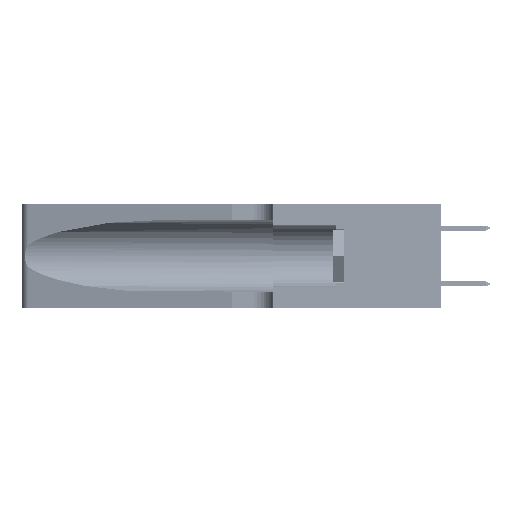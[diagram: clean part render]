
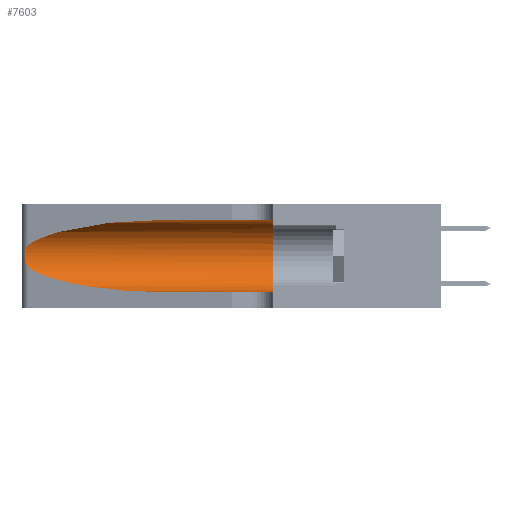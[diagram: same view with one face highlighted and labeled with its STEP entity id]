
A CAD part, left-side view. The second image highlights one B-rep face of the part: STEP entity #7603.
In plain terms, the highlighted cylindrical face has radius 3.308 mm (diameter 6.617 mm), a partial arc.
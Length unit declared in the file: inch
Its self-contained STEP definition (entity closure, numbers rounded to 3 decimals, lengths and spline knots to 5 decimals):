
#663 = EDGE_CURVE ( 'NONE', #46274, #41086, #32545, .T. ) ;
#688 = VERTEX_POINT ( 'NONE', #49093 ) ;
#1128 = VECTOR ( 'NONE', #25476, 39.37008 ) ;
#1929 = CIRCLE ( 'NONE', #25278, 0.13025 ) ;
#2452 = ORIENTED_EDGE ( 'NONE', *, *, #33223, .T. ) ;
#2750 = CARTESIAN_POINT ( 'NONE',  ( 0.18966, 0.96281, 0.05475 ) ) ;
#3899 = CARTESIAN_POINT ( 'NONE',  ( 0.25487, 1.22718, 0.14631 ) ) ;
#6075 = DIRECTION ( 'NONE',  ( 0., 0., -1. ) ) ;
#6347 = CARTESIAN_POINT ( 'NONE',  ( 0.1305, 1.61858, 0.31525 ) ) ;
#7603 = ADVANCED_FACE ( 'NONE', ( #39147 ), #17795, .F. ) ;
#7641 = CARTESIAN_POINT ( 'NONE',  ( 0.25639, 1.23184, 0.21858 ) ) ;
#9810 = CARTESIAN_POINT ( 'NONE',  ( 0.1305, 1.61858, 0.185 ) ) ;
#9812 = EDGE_CURVE ( 'NONE', #41086, #22904, #37721, .T. ) ;
#10245 = VECTOR ( 'NONE', #31452, 39.37008 ) ;
#11208 =( BOUNDED_CURVE ( )  B_SPLINE_CURVE ( 3, ( #37047, #29460, #2750, #29626 ),
 .UNSPECIFIED., .F., .T. ) 
 B_SPLINE_CURVE_WITH_KNOTS ( ( 4, 4 ),
 ( 3.44316, 4.71239 ),
 .UNSPECIFIED. ) 
 CURVE ( )  GEOMETRIC_REPRESENTATION_ITEM ( )  RATIONAL_B_SPLINE_CURVE ( ( 1., 0.87, 0.87, 1. ) ) 
 REPRESENTATION_ITEM ( '' )  );
#11456 = LINE ( 'NONE', #6347, #10245 ) ;
#11561 = CARTESIAN_POINT ( 'NONE',  ( 0.25854, 1.2359, 0.20912 ) ) ;
#12091 = ORIENTED_EDGE ( 'NONE', *, *, #32226, .F. ) ;
#14748 = CARTESIAN_POINT ( 'NONE',  ( 0.18966, 0.96281, 0.31525 ) ) ;
#14938 = EDGE_CURVE ( 'NONE', #22904, #42205, #11208, .T. ) ;
#15421 = CARTESIAN_POINT ( 'NONE',  ( 0.26075, 1.23896, 0.19203 ) ) ;
#15796 = ORIENTED_EDGE ( 'NONE', *, *, #663, .T. ) ;
#15965 = ORIENTED_EDGE ( 'NONE', *, *, #44763, .F. ) ;
#16030 = CARTESIAN_POINT ( 'NONE',  ( 0.25487, 1.22718, 0.22369 ) ) ;
#17795 = CYLINDRICAL_SURFACE ( 'NONE', #43287, 0.13025 ) ;
#18470 = CARTESIAN_POINT ( 'NONE',  ( 0.25487, 1.22718, 0.14631 ) ) ;
#19280 = CARTESIAN_POINT ( 'NONE',  ( 0.1305, 0.35, 0.185 ) ) ;
#19292 = CARTESIAN_POINT ( 'NONE',  ( 0.26017, 1.23833, 0.17102 ) ) ;
#21744 = LINE ( 'NONE', #36719, #1128 ) ;
#22904 = VERTEX_POINT ( 'NONE', #18470 ) ;
#23091 = DIRECTION ( 'NONE',  ( 0., 0., 1. ) ) ;
#23106 = CARTESIAN_POINT ( 'NONE',  ( 0.25789, 1.23486, 0.15765 ) ) ;
#24082 = CARTESIAN_POINT ( 'NONE',  ( 0.1305, 0.72297, 0.31525 ) ) ;
#25278 = AXIS2_PLACEMENT_3D ( 'NONE', #19280, #45752, #23091 ) ;
#25476 = DIRECTION ( 'NONE',  ( 0., -1., 0. ) ) ;
#26249 = CARTESIAN_POINT ( 'NONE',  ( 0.2373, 1.15595, 0.28018 ) ) ;
#26694 = ORIENTED_EDGE ( 'NONE', *, *, #9812, .T. ) ;
#26910 = CARTESIAN_POINT ( 'NONE',  ( 0.25555, 1.22993, 0.14849 ) ) ;
#29008 = DIRECTION ( 'NONE',  ( 0., -1., 0. ) ) ;
#29460 = CARTESIAN_POINT ( 'NONE',  ( 0.2373, 1.15595, 0.08982 ) ) ;
#29626 = CARTESIAN_POINT ( 'NONE',  ( 0.1305, 0.72297, 0.05475 ) ) ;
#30057 = CARTESIAN_POINT ( 'NONE',  ( 0.25487, 1.22718, 0.22369 ) ) ;
#31452 = DIRECTION ( 'NONE',  ( 0., -1., 0. ) ) ;
#32226 = EDGE_CURVE ( 'NONE', #44351, #688, #1929, .T. ) ;
#32322 = CARTESIAN_POINT ( 'NONE',  ( 0.1305, 0.72297, 0.05475 ) ) ;
#32545 =( BOUNDED_CURVE ( )  B_SPLINE_CURVE ( 3, ( #45101, #14748, #26249, #30057 ),
 .UNSPECIFIED., .F., .T. ) 
 B_SPLINE_CURVE_WITH_KNOTS ( ( 4, 4 ),
 ( 1.5708, 2.84003 ),
 .UNSPECIFIED. ) 
 CURVE ( )  GEOMETRIC_REPRESENTATION_ITEM ( )  RATIONAL_B_SPLINE_CURVE ( ( 1., 0.87, 0.87, 1. ) ) 
 REPRESENTATION_ITEM ( '' )  );
#33223 = EDGE_CURVE ( 'NONE', #42205, #688, #21744, .T. ) ;
#34332 = CARTESIAN_POINT ( 'NONE',  ( 0.25787, 1.23484, 0.2124 ) ) ;
#36719 = CARTESIAN_POINT ( 'NONE',  ( 0.1305, 1.61858, 0.05475 ) ) ;
#37047 = CARTESIAN_POINT ( 'NONE',  ( 0.25487, 1.22718, 0.14631 ) ) ;
#37307 = ORIENTED_EDGE ( 'NONE', *, *, #14938, .T. ) ;
#37465 = CARTESIAN_POINT ( 'NONE',  ( 0.1305, 0.35, 0.31525 ) ) ;
#37630 = CARTESIAN_POINT ( 'NONE',  ( 0.25639, 1.23186, 0.15144 ) ) ;
#37721 = B_SPLINE_CURVE_WITH_KNOTS ( 'NONE', 3,
 ( #49425, #37991, #7641, #34332, #11561, #38161, #15421, #41971, #19292, #45762, #23106, #37630, #26910, #3899 ),
 .UNSPECIFIED., .F., .F.,
 ( 4, 2, 2, 2, 2, 2, 4 ),
 ( 0., 0.00027, 0.00053, 0.00107, 0.0016, 0.00187, 0.00214 ),
 .UNSPECIFIED. ) ;
#37991 = CARTESIAN_POINT ( 'NONE',  ( 0.25555, 1.22994, 0.2215 ) ) ;
#38161 = CARTESIAN_POINT ( 'NONE',  ( 0.26018, 1.23835, 0.19895 ) ) ;
#38562 = EDGE_LOOP ( 'NONE', ( #15796, #26694, #37307, #2452, #12091, #15965 ) ) ;
#39147 = FACE_OUTER_BOUND ( 'NONE', #38562, .T. ) ;
#41086 = VERTEX_POINT ( 'NONE', #16030 ) ;
#41971 = CARTESIAN_POINT ( 'NONE',  ( 0.26075, 1.23896, 0.178 ) ) ;
#42205 = VERTEX_POINT ( 'NONE', #32322 ) ;
#43287 = AXIS2_PLACEMENT_3D ( 'NONE', #9810, #29008, #6075 ) ;
#44351 = VERTEX_POINT ( 'NONE', #37465 ) ;
#44763 = EDGE_CURVE ( 'NONE', #46274, #44351, #11456, .T. ) ;
#45101 = CARTESIAN_POINT ( 'NONE',  ( 0.1305, 0.72297, 0.31525 ) ) ;
#45752 = DIRECTION ( 'NONE',  ( 0., 1., 0. ) ) ;
#45762 = CARTESIAN_POINT ( 'NONE',  ( 0.25856, 1.23593, 0.16098 ) ) ;
#46274 = VERTEX_POINT ( 'NONE', #24082 ) ;
#49093 = CARTESIAN_POINT ( 'NONE',  ( 0.1305, 0.35, 0.05475 ) ) ;
#49425 = CARTESIAN_POINT ( 'NONE',  ( 0.25487, 1.22718, 0.22369 ) ) ;
